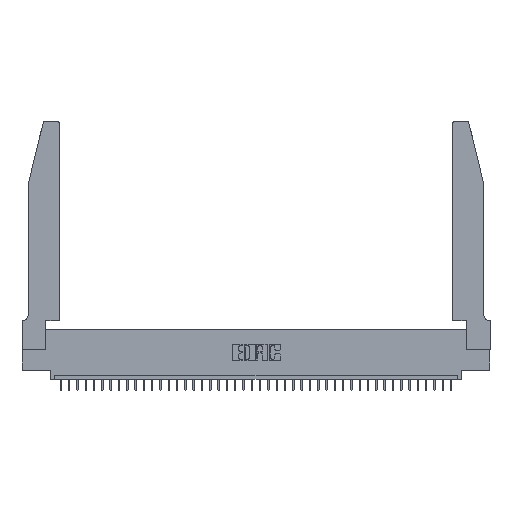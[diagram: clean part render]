
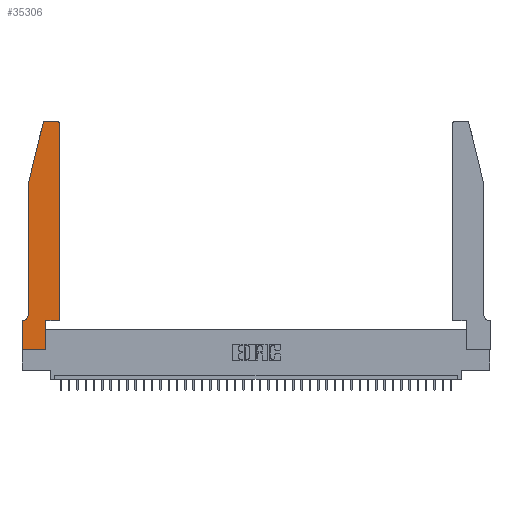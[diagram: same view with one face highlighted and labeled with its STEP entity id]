
A CAD part, top view. The second image highlights one B-rep face of the part: STEP entity #35306.
In plain terms, the highlighted planar face has unit normal (0, 0, 1).
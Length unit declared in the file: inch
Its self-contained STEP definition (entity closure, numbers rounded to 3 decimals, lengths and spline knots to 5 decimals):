
#34 = DIRECTION ( 'NONE',  ( 0., 0., -1. ) ) ;
#918 = VERTEX_POINT ( 'NONE', #36547 ) ;
#2266 = CARTESIAN_POINT ( 'NONE',  ( 0.2865, 0.35, 0.37 ) ) ;
#3426 = VECTOR ( 'NONE', #3623, 39.37008 ) ;
#3623 = DIRECTION ( 'NONE',  ( -1., 0., 0. ) ) ;
#3974 = DIRECTION ( 'NONE',  ( -1., 0., 0. ) ) ;
#4304 = CIRCLE ( 'NONE', #17298, 0.03 ) ;
#4353 = FACE_OUTER_BOUND ( 'NONE', #6482, .T. ) ;
#4975 = ORIENTED_EDGE ( 'NONE', *, *, #16616, .T. ) ;
#5420 = DIRECTION ( 'NONE',  ( 1., 0., 0. ) ) ;
#5497 = DIRECTION ( 'NONE',  ( 1., 0., 0. ) ) ;
#5721 = ORIENTED_EDGE ( 'NONE', *, *, #12452, .T. ) ;
#5735 = CARTESIAN_POINT ( 'NONE',  ( 0., 0., 0.37 ) ) ;
#5811 = CARTESIAN_POINT ( 'NONE',  ( 0.4205, 2.72, 0.37 ) ) ;
#6414 = AXIS2_PLACEMENT_3D ( 'NONE', #9870, #10265, #34694 ) ;
#6476 = ORIENTED_EDGE ( 'NONE', *, *, #38782, .T. ) ;
#6482 = EDGE_LOOP ( 'NONE', ( #34910, #4975, #29750, #8872, #18944, #6476, #26919, #7471, #36484, #34275, #21085, #5721 ) ) ;
#7302 = VERTEX_POINT ( 'NONE', #22407 ) ;
#7471 = ORIENTED_EDGE ( 'NONE', *, *, #31872, .T. ) ;
#7542 = CARTESIAN_POINT ( 'NONE',  ( 0.0755, 2., 0.37 ) ) ;
#8872 = ORIENTED_EDGE ( 'NONE', *, *, #38491, .T. ) ;
#9142 = DIRECTION ( 'NONE',  ( 1., 0., 0. ) ) ;
#9384 = EDGE_CURVE ( 'NONE', #23903, #10816, #29870, .T. ) ;
#9582 = VERTEX_POINT ( 'NONE', #32026 ) ;
#9870 = CARTESIAN_POINT ( 'NONE',  ( 0., 0.35, 0.37 ) ) ;
#10265 = DIRECTION ( 'NONE',  ( 0., 0., 1. ) ) ;
#10470 = EDGE_CURVE ( 'NONE', #27434, #22249, #32270, .T. ) ;
#10816 = VERTEX_POINT ( 'NONE', #26337 ) ;
#11419 = EDGE_CURVE ( 'NONE', #33403, #18491, #15440, .T. ) ;
#12452 = EDGE_CURVE ( 'NONE', #21742, #33403, #28132, .T. ) ;
#12841 = CARTESIAN_POINT ( 'NONE',  ( 0.2865, 0., 0.37 ) ) ;
#13944 = VECTOR ( 'NONE', #15422, 39.37008 ) ;
#15422 = DIRECTION ( 'NONE',  ( 0., 1., 0. ) ) ;
#15440 = LINE ( 'NONE', #15650, #3426 ) ;
#15650 = CARTESIAN_POINT ( 'NONE',  ( 0.2605, 2.75, 0.37 ) ) ;
#15685 = VECTOR ( 'NONE', #17608, 39.37008 ) ;
#16427 = VERTEX_POINT ( 'NONE', #12841 ) ;
#16616 = EDGE_CURVE ( 'NONE', #18491, #918, #4304, .T. ) ;
#16670 = CARTESIAN_POINT ( 'NONE',  ( 0.4505, 2.72, 0.37 ) ) ;
#17298 = AXIS2_PLACEMENT_3D ( 'NONE', #27488, #33379, #9142 ) ;
#17319 = CARTESIAN_POINT ( 'NONE',  ( 0., 0., 0.37 ) ) ;
#17608 = DIRECTION ( 'NONE',  ( 1., 0., 0. ) ) ;
#18027 = EDGE_CURVE ( 'NONE', #25563, #7302, #30398, .T. ) ;
#18362 = DIRECTION ( 'NONE',  ( 0., 1., 0. ) ) ;
#18491 = VERTEX_POINT ( 'NONE', #34931 ) ;
#18944 = ORIENTED_EDGE ( 'NONE', *, *, #9384, .T. ) ;
#19497 = VECTOR ( 'NONE', #3974, 39.37008 ) ;
#19774 = CARTESIAN_POINT ( 'NONE',  ( 0.0755, 0.42, 0.37 ) ) ;
#21030 = DIRECTION ( 'NONE',  ( 0., -1., 0. ) ) ;
#21085 = ORIENTED_EDGE ( 'NONE', *, *, #28577, .T. ) ;
#21154 = CARTESIAN_POINT ( 'NONE',  ( 0.4505, 0.35, 0.37 ) ) ;
#21742 = VERTEX_POINT ( 'NONE', #16670 ) ;
#22051 = AXIS2_PLACEMENT_3D ( 'NONE', #28180, #34, #22258 ) ;
#22249 = VERTEX_POINT ( 'NONE', #34637 ) ;
#22258 = DIRECTION ( 'NONE',  ( -1., 0., 0. ) ) ;
#22407 = CARTESIAN_POINT ( 'NONE',  ( 0., 0., 0.37 ) ) ;
#22606 = CARTESIAN_POINT ( 'NONE',  ( 0.2865, 0.35, 0.37 ) ) ;
#23567 = AXIS2_PLACEMENT_3D ( 'NONE', #5811, #30670, #5420 ) ;
#23645 = DIRECTION ( 'NONE',  ( 0., -1., 0. ) ) ;
#23903 = VERTEX_POINT ( 'NONE', #19774 ) ;
#25563 = VERTEX_POINT ( 'NONE', #28319 ) ;
#25592 = LINE ( 'NONE', #38015, #19497 ) ;
#25649 = CARTESIAN_POINT ( 'NONE',  ( 0.4205, 2.75, 0.37 ) ) ;
#25853 = VECTOR ( 'NONE', #5497, 39.37008 ) ;
#25898 = CARTESIAN_POINT ( 'NONE',  ( 0.0755, 2., 0.37 ) ) ;
#26337 = CARTESIAN_POINT ( 'NONE',  ( 0.0055, 0.35, 0.37 ) ) ;
#26919 = ORIENTED_EDGE ( 'NONE', *, *, #18027, .T. ) ;
#27434 = VERTEX_POINT ( 'NONE', #22606 ) ;
#27488 = CARTESIAN_POINT ( 'NONE',  ( 0.284, 2.72, 0.37 ) ) ;
#27763 = VECTOR ( 'NONE', #21030, 39.37008 ) ;
#28132 = CIRCLE ( 'NONE', #23567, 0.03 ) ;
#28180 = CARTESIAN_POINT ( 'NONE',  ( 0.0055, 0.42, 0.37 ) ) ;
#28319 = CARTESIAN_POINT ( 'NONE',  ( 0., 0.35, 0.37 ) ) ;
#28577 = EDGE_CURVE ( 'NONE', #22249, #21742, #39687, .T. ) ;
#28951 = LINE ( 'NONE', #25898, #38971 ) ;
#29750 = ORIENTED_EDGE ( 'NONE', *, *, #38276, .T. ) ;
#29870 = CIRCLE ( 'NONE', #22051, 0.07 ) ;
#30398 = LINE ( 'NONE', #5735, #27763 ) ;
#30670 = DIRECTION ( 'NONE',  ( 0., 0., 1. ) ) ;
#31180 = VECTOR ( 'NONE', #23645, 39.37008 ) ;
#31872 = EDGE_CURVE ( 'NONE', #7302, #16427, #39313, .T. ) ;
#32026 = CARTESIAN_POINT ( 'NONE',  ( 0.0755, 2., 0.37 ) ) ;
#32270 = LINE ( 'NONE', #38990, #15685 ) ;
#32610 = EDGE_CURVE ( 'NONE', #16427, #27434, #39758, .T. ) ;
#33017 = VECTOR ( 'NONE', #18362, 39.37008 ) ;
#33379 = DIRECTION ( 'NONE',  ( 0., 0., 1. ) ) ;
#33403 = VERTEX_POINT ( 'NONE', #25649 ) ;
#34275 = ORIENTED_EDGE ( 'NONE', *, *, #10470, .T. ) ;
#34637 = CARTESIAN_POINT ( 'NONE',  ( 0.4505, 0.35, 0.37 ) ) ;
#34694 = DIRECTION ( 'NONE',  ( 1., 0., 0. ) ) ;
#34910 = ORIENTED_EDGE ( 'NONE', *, *, #11419, .T. ) ;
#34931 = CARTESIAN_POINT ( 'NONE',  ( 0.284, 2.75, 0.37 ) ) ;
#35306 = ADVANCED_FACE ( 'NONE', ( #4353 ), #38175, .T. ) ;
#36484 = ORIENTED_EDGE ( 'NONE', *, *, #32610, .T. ) ;
#36547 = CARTESIAN_POINT ( 'NONE',  ( 0.25487, 2.72718, 0.37 ) ) ;
#38015 = CARTESIAN_POINT ( 'NONE',  ( 0.0755, 0.35, 0.37 ) ) ;
#38175 = PLANE ( 'NONE',  #6414 ) ;
#38276 = EDGE_CURVE ( 'NONE', #918, #9582, #28951, .T. ) ;
#38310 = DIRECTION ( 'NONE',  ( -0.239, -0.971, 0. ) ) ;
#38491 = EDGE_CURVE ( 'NONE', #9582, #23903, #39315, .T. ) ;
#38782 = EDGE_CURVE ( 'NONE', #10816, #25563, #25592, .T. ) ;
#38971 = VECTOR ( 'NONE', #38310, 39.37008 ) ;
#38990 = CARTESIAN_POINT ( 'NONE',  ( 0.4505, 0.35, 0.37 ) ) ;
#39313 = LINE ( 'NONE', #17319, #25853 ) ;
#39315 = LINE ( 'NONE', #7542, #31180 ) ;
#39687 = LINE ( 'NONE', #21154, #13944 ) ;
#39758 = LINE ( 'NONE', #2266, #33017 ) ;
